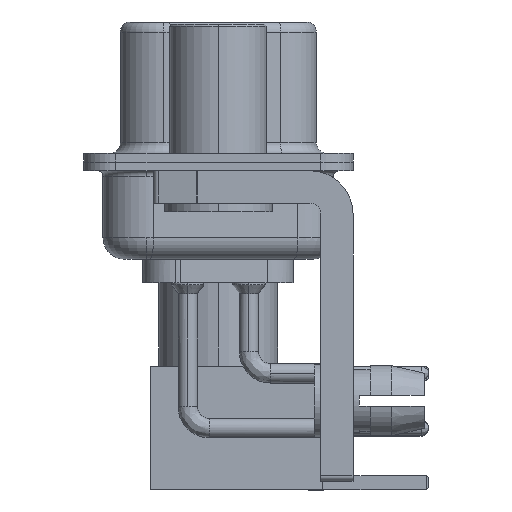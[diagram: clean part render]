
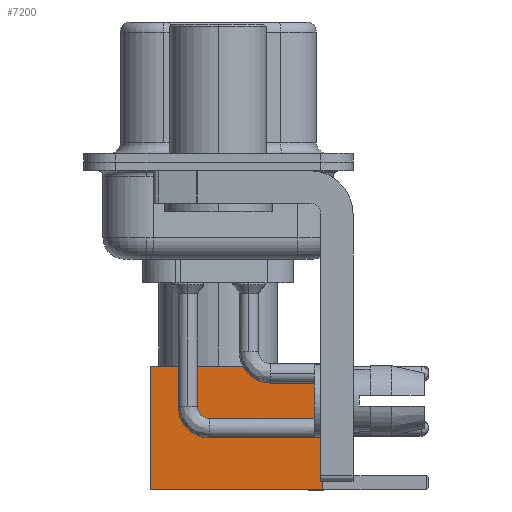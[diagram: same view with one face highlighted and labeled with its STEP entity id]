
A CAD part, left-side view. The second image highlights one B-rep face of the part: STEP entity #7200.
In plain terms, the highlighted face is planar.
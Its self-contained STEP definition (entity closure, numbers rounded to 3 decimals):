
#729 = AXIS2_PLACEMENT_3D ( 'NONE', #15438, #33807, #28826 ) ;
#4132 = CARTESIAN_POINT ( 'NONE',  ( 0., 2.875, 0. ) ) ;
#4256 = VERTEX_POINT ( 'NONE', #24560 ) ;
#4760 = VERTEX_POINT ( 'NONE', #25198 ) ;
#7200 = ADVANCED_FACE ( 'NONE', ( #8025 ), #26079, .T. ) ;
#7273 = VECTOR ( 'NONE', #16860, 1000. ) ;
#7671 = VECTOR ( 'NONE', #11274, 1000. ) ;
#7805 = EDGE_CURVE ( 'NONE', #4256, #9533, #24264, .T. ) ;
#8025 = FACE_OUTER_BOUND ( 'NONE', #33706, .T. ) ;
#8363 = LINE ( 'NONE', #27265, #7671 ) ;
#9533 = VERTEX_POINT ( 'NONE', #29812 ) ;
#11274 = DIRECTION ( 'NONE',  ( 0., 0., -1. ) ) ;
#14355 = ORIENTED_EDGE ( 'NONE', *, *, #17338, .T. ) ;
#15438 = CARTESIAN_POINT ( 'NONE',  ( 2.875, 2.875, 0. ) ) ;
#16700 = VERTEX_POINT ( 'NONE', #17343 ) ;
#16860 = DIRECTION ( 'NONE',  ( -1., 0., 0. ) ) ;
#17194 = LINE ( 'NONE', #4132, #30099 ) ;
#17338 = EDGE_CURVE ( 'NONE', #4760, #16700, #17194, .T. ) ;
#17343 = CARTESIAN_POINT ( 'NONE',  ( -2.875, 2.875, 0. ) ) ;
#18348 = EDGE_CURVE ( 'NONE', #4256, #4760, #8363, .T. ) ;
#21084 = VECTOR ( 'NONE', #21424, 1000. ) ;
#21424 = DIRECTION ( 'NONE',  ( 0., 0., -1. ) ) ;
#21827 = ORIENTED_EDGE ( 'NONE', *, *, #18348, .T. ) ;
#22021 = CARTESIAN_POINT ( 'NONE',  ( 0., 2.875, 8. ) ) ;
#23167 = CARTESIAN_POINT ( 'NONE',  ( -2.875, 2.875, 0. ) ) ;
#23795 = DIRECTION ( 'NONE',  ( -1., 0., 0. ) ) ;
#23976 = ORIENTED_EDGE ( 'NONE', *, *, #7805, .F. ) ;
#23983 = ORIENTED_EDGE ( 'NONE', *, *, #33994, .F. ) ;
#24264 = LINE ( 'NONE', #22021, #7273 ) ;
#24560 = CARTESIAN_POINT ( 'NONE',  ( 2.875, 2.875, 8. ) ) ;
#25198 = CARTESIAN_POINT ( 'NONE',  ( 2.875, 2.875, 0. ) ) ;
#26079 = PLANE ( 'NONE',  #729 ) ;
#27265 = CARTESIAN_POINT ( 'NONE',  ( 2.875, 2.875, 0. ) ) ;
#28317 = LINE ( 'NONE', #23167, #21084 ) ;
#28826 = DIRECTION ( 'NONE',  ( 0., 0., 1. ) ) ;
#29812 = CARTESIAN_POINT ( 'NONE',  ( -2.875, 2.875, 8. ) ) ;
#30099 = VECTOR ( 'NONE', #23795, 1000. ) ;
#33706 = EDGE_LOOP ( 'NONE', ( #21827, #14355, #23983, #23976 ) ) ;
#33807 = DIRECTION ( 'NONE',  ( 0., 1., 0. ) ) ;
#33994 = EDGE_CURVE ( 'NONE', #9533, #16700, #28317, .T. ) ;
